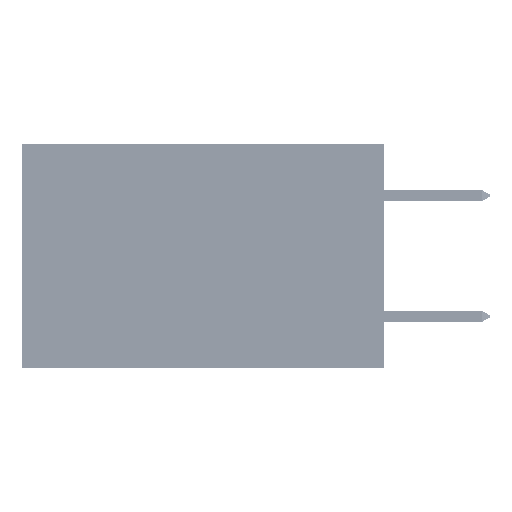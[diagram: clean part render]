
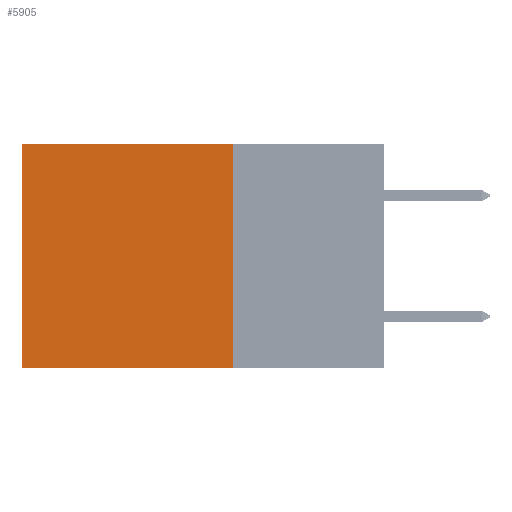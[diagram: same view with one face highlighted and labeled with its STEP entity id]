
A CAD part, left-side view. The second image highlights one B-rep face of the part: STEP entity #5905.
In plain terms, the highlighted planar face has unit normal (-1, 0, 0).
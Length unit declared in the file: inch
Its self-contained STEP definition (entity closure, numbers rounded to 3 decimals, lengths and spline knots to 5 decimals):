
#2014 = DIRECTION ( 'NONE',  ( 0., 0., -1. ) ) ;
#2457 = CARTESIAN_POINT ( 'NONE',  ( 0.2875, 0.25, -0.37 ) ) ;
#3213 = ORIENTED_EDGE ( 'NONE', *, *, #7920, .T. ) ;
#4508 = CARTESIAN_POINT ( 'NONE',  ( 0.2875, 0.6, 0. ) ) ;
#4866 = VERTEX_POINT ( 'NONE', #6756 ) ;
#5905 = ADVANCED_FACE ( 'NONE', ( #38795 ), #34724, .F. ) ;
#6425 = CARTESIAN_POINT ( 'NONE',  ( 0.2875, 0.25, 0. ) ) ;
#6739 = EDGE_LOOP ( 'NONE', ( #3213, #42982, #31456, #40388 ) ) ;
#6756 = CARTESIAN_POINT ( 'NONE',  ( 0.2875, 0.6, -0.37 ) ) ;
#7920 = EDGE_CURVE ( 'NONE', #17680, #4866, #24842, .T. ) ;
#10566 = VECTOR ( 'NONE', #13766, 39.37008 ) ;
#12081 = VECTOR ( 'NONE', #33443, 39.37008 ) ;
#13766 = DIRECTION ( 'NONE',  ( 0., 0., -1. ) ) ;
#14037 = VECTOR ( 'NONE', #18393, 39.37008 ) ;
#16272 = VERTEX_POINT ( 'NONE', #2457 ) ;
#17680 = VERTEX_POINT ( 'NONE', #4508 ) ;
#18393 = DIRECTION ( 'NONE',  ( 0., 0., -1. ) ) ;
#18887 = CARTESIAN_POINT ( 'NONE',  ( 0.2875, 0.25, -0.37 ) ) ;
#19358 = CARTESIAN_POINT ( 'NONE',  ( 0.2875, 0.25, 0. ) ) ;
#20404 = CARTESIAN_POINT ( 'NONE',  ( 0.2875, 0.25, 0. ) ) ;
#20926 = LINE ( 'NONE', #19358, #32923 ) ;
#24842 = LINE ( 'NONE', #47066, #14037 ) ;
#25195 = CARTESIAN_POINT ( 'NONE',  ( 0.2875, 0.25, 0. ) ) ;
#26977 = DIRECTION ( 'NONE',  ( 0., 1., 0. ) ) ;
#28771 = VERTEX_POINT ( 'NONE', #6425 ) ;
#31456 = ORIENTED_EDGE ( 'NONE', *, *, #34582, .F. ) ;
#32923 = VECTOR ( 'NONE', #26977, 39.37008 ) ;
#33443 = DIRECTION ( 'NONE',  ( 0., 1., 0. ) ) ;
#34582 = EDGE_CURVE ( 'NONE', #28771, #16272, #42683, .T. ) ;
#34724 = PLANE ( 'NONE',  #45560 ) ;
#37146 = EDGE_CURVE ( 'NONE', #28771, #17680, #20926, .T. ) ;
#38795 = FACE_OUTER_BOUND ( 'NONE', #6739, .T. ) ;
#40388 = ORIENTED_EDGE ( 'NONE', *, *, #37146, .T. ) ;
#42683 = LINE ( 'NONE', #25195, #10566 ) ;
#42982 = ORIENTED_EDGE ( 'NONE', *, *, #46312, .F. ) ;
#43508 = LINE ( 'NONE', #18887, #12081 ) ;
#45560 = AXIS2_PLACEMENT_3D ( 'NONE', #20404, #46643, #2014 ) ;
#46312 = EDGE_CURVE ( 'NONE', #16272, #4866, #43508, .T. ) ;
#46643 = DIRECTION ( 'NONE',  ( 1., 0., 0. ) ) ;
#47066 = CARTESIAN_POINT ( 'NONE',  ( 0.2875, 0.6, 0. ) ) ;
